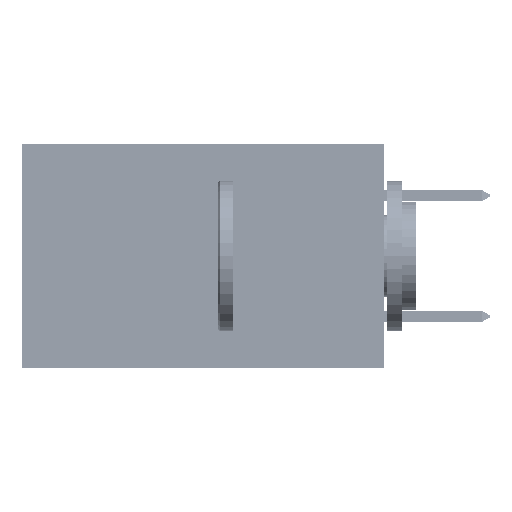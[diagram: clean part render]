
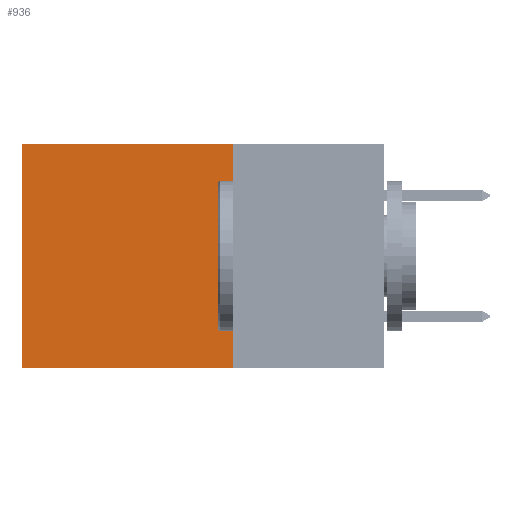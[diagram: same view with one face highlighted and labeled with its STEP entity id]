
A CAD part, left-side view. The second image highlights one B-rep face of the part: STEP entity #936.
In plain terms, the highlighted planar face has unit normal (-1, 0, 0).
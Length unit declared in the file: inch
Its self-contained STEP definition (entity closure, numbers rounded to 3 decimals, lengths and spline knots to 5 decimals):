
#120 = EDGE_CURVE ( 'NONE', #24101, #11989, #31438, .T. ) ;
#775 = VECTOR ( 'NONE', #973, 39.37008 ) ;
#936 = ADVANCED_FACE ( 'NONE', ( #49647 ), #8411, .F. ) ;
#973 = DIRECTION ( 'NONE',  ( 0., 0., -1. ) ) ;
#4391 = DIRECTION ( 'NONE',  ( 1., 0., 0. ) ) ;
#5463 = CARTESIAN_POINT ( 'NONE',  ( 0.2875, 0.25, -0.37 ) ) ;
#8292 = LINE ( 'NONE', #45149, #775 ) ;
#8411 = PLANE ( 'NONE',  #29198 ) ;
#11989 = VERTEX_POINT ( 'NONE', #41837 ) ;
#12038 = LINE ( 'NONE', #48400, #15825 ) ;
#13291 = EDGE_CURVE ( 'NONE', #11989, #36701, #8292, .T. ) ;
#14181 = CARTESIAN_POINT ( 'NONE',  ( 0.2875, 0.25, -0.37 ) ) ;
#15546 = VECTOR ( 'NONE', #33533, 39.37008 ) ;
#15825 = VECTOR ( 'NONE', #28609, 39.37008 ) ;
#17989 = ORIENTED_EDGE ( 'NONE', *, *, #27717, .F. ) ;
#19203 = EDGE_CURVE ( 'NONE', #39142, #36701, #35629, .T. ) ;
#24101 = VERTEX_POINT ( 'NONE', #47589 ) ;
#24501 = VECTOR ( 'NONE', #41833, 39.37008 ) ;
#24881 = DIRECTION ( 'NONE',  ( 0., 0., -1. ) ) ;
#27717 = EDGE_CURVE ( 'NONE', #24101, #39142, #12038, .T. ) ;
#28609 = DIRECTION ( 'NONE',  ( 0., 0., -1. ) ) ;
#28766 = CARTESIAN_POINT ( 'NONE',  ( 0.2875, 0.25, 0. ) ) ;
#29198 = AXIS2_PLACEMENT_3D ( 'NONE', #28766, #4391, #24881 ) ;
#31438 = LINE ( 'NONE', #37820, #24501 ) ;
#33533 = DIRECTION ( 'NONE',  ( 0., 1., 0. ) ) ;
#35629 = LINE ( 'NONE', #5463, #15546 ) ;
#36701 = VERTEX_POINT ( 'NONE', #43967 ) ;
#36781 = ORIENTED_EDGE ( 'NONE', *, *, #13291, .T. ) ;
#37820 = CARTESIAN_POINT ( 'NONE',  ( 0.2875, 0.25, 0. ) ) ;
#38861 = EDGE_LOOP ( 'NONE', ( #36781, #47037, #17989, #42855 ) ) ;
#39142 = VERTEX_POINT ( 'NONE', #14181 ) ;
#41833 = DIRECTION ( 'NONE',  ( 0., 1., 0. ) ) ;
#41837 = CARTESIAN_POINT ( 'NONE',  ( 0.2875, 0.6, 0. ) ) ;
#42855 = ORIENTED_EDGE ( 'NONE', *, *, #120, .T. ) ;
#43967 = CARTESIAN_POINT ( 'NONE',  ( 0.2875, 0.6, -0.37 ) ) ;
#45149 = CARTESIAN_POINT ( 'NONE',  ( 0.2875, 0.6, 0. ) ) ;
#47037 = ORIENTED_EDGE ( 'NONE', *, *, #19203, .F. ) ;
#47589 = CARTESIAN_POINT ( 'NONE',  ( 0.2875, 0.25, 0. ) ) ;
#48400 = CARTESIAN_POINT ( 'NONE',  ( 0.2875, 0.25, 0. ) ) ;
#49647 = FACE_OUTER_BOUND ( 'NONE', #38861, .T. ) ;
